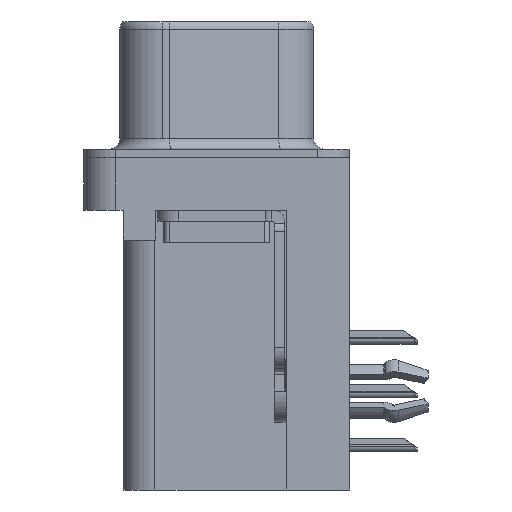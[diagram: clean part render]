
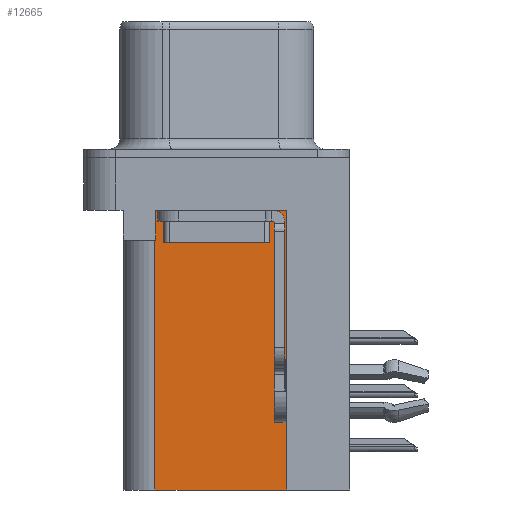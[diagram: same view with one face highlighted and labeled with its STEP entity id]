
A CAD part, left-side view. The second image highlights one B-rep face of the part: STEP entity #12665.
In plain terms, the highlighted planar face has unit normal (-1, 0, 0).
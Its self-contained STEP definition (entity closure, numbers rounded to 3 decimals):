
#93 = VECTOR ( 'NONE', #17923, 1000. ) ;
#314 = DIRECTION ( 'NONE',  ( 0., 0., 1. ) ) ;
#1641 = CARTESIAN_POINT ( 'NONE',  ( 3.7, 2.895, -3.9 ) ) ;
#2172 = VERTEX_POINT ( 'NONE', #4198 ) ;
#2786 = EDGE_CURVE ( 'NONE', #2172, #5257, #12546, .T. ) ;
#2796 = VECTOR ( 'NONE', #14160, 1000. ) ;
#2877 = LINE ( 'NONE', #1641, #2796 ) ;
#3322 = EDGE_CURVE ( 'NONE', #7064, #2172, #9905, .T. ) ;
#3385 = EDGE_CURVE ( 'NONE', #7064, #19916, #9599, .T. ) ;
#4198 = CARTESIAN_POINT ( 'NONE',  ( 3.7, 2.925, -15.7 ) ) ;
#4380 = DIRECTION ( 'NONE',  ( 0., 1., 0. ) ) ;
#5216 = ORIENTED_EDGE ( 'NONE', *, *, #24734, .T. ) ;
#5257 = VERTEX_POINT ( 'NONE', #14286 ) ;
#5856 = FACE_OUTER_BOUND ( 'NONE', #13048, .T. ) ;
#7064 = VERTEX_POINT ( 'NONE', #27423 ) ;
#9599 = LINE ( 'NONE', #19810, #9662 ) ;
#9662 = VECTOR ( 'NONE', #314, 1000. ) ;
#9745 = VECTOR ( 'NONE', #4380, 1000. ) ;
#9905 = LINE ( 'NONE', #25027, #9745 ) ;
#11982 = VECTOR ( 'NONE', #12486, 1000. ) ;
#12486 = DIRECTION ( 'NONE',  ( 0., 1., 0. ) ) ;
#12515 = VECTOR ( 'NONE', #23808, 1000. ) ;
#12546 = LINE ( 'NONE', #25858, #12515 ) ;
#12619 = LINE ( 'NONE', #17079, #11982 ) ;
#12665 = ADVANCED_FACE ( 'NONE', ( #5856 ), #21833, .F. ) ;
#13048 = EDGE_LOOP ( 'NONE', ( #30845, #30718, #5216, #14829, #28583, #13644 ) ) ;
#13597 = LINE ( 'NONE', #15676, #93 ) ;
#13644 = ORIENTED_EDGE ( 'NONE', *, *, #3385, .T. ) ;
#13768 = CARTESIAN_POINT ( 'NONE',  ( 3.7, -3.295, -2.5 ) ) ;
#14160 = DIRECTION ( 'NONE',  ( 0., 0., -1. ) ) ;
#14286 = CARTESIAN_POINT ( 'NONE',  ( 3.7, 2.925, -3.9 ) ) ;
#14829 = ORIENTED_EDGE ( 'NONE', *, *, #2786, .F. ) ;
#14872 = CARTESIAN_POINT ( 'NONE',  ( 3.7, -3.295, -15.7 ) ) ;
#15676 = CARTESIAN_POINT ( 'NONE',  ( 3.7, 0., -3.9 ) ) ;
#16013 = VERTEX_POINT ( 'NONE', #27920 ) ;
#17079 = CARTESIAN_POINT ( 'NONE',  ( 3.7, -3.295, -2.5 ) ) ;
#17171 = DIRECTION ( 'NONE',  ( 0., 0., -1. ) ) ;
#17923 = DIRECTION ( 'NONE',  ( 0., 1., 0. ) ) ;
#18250 = VERTEX_POINT ( 'NONE', #21418 ) ;
#18843 = EDGE_CURVE ( 'NONE', #19916, #18250, #12619, .T. ) ;
#19810 = CARTESIAN_POINT ( 'NONE',  ( 3.7, -3.295, -15.7 ) ) ;
#19916 = VERTEX_POINT ( 'NONE', #13768 ) ;
#19984 = EDGE_CURVE ( 'NONE', #18250, #16013, #2877, .T. ) ;
#21418 = CARTESIAN_POINT ( 'NONE',  ( 3.7, 2.895, -2.5 ) ) ;
#21833 = PLANE ( 'NONE',  #22133 ) ;
#22133 = AXIS2_PLACEMENT_3D ( 'NONE', #14872, #31141, #17171 ) ;
#23808 = DIRECTION ( 'NONE',  ( 0., 0., 1. ) ) ;
#24734 = EDGE_CURVE ( 'NONE', #16013, #5257, #13597, .T. ) ;
#25027 = CARTESIAN_POINT ( 'NONE',  ( 3.7, -3.295, -15.7 ) ) ;
#25858 = CARTESIAN_POINT ( 'NONE',  ( 3.7, 2.925, -15.7 ) ) ;
#27423 = CARTESIAN_POINT ( 'NONE',  ( 3.7, -3.295, -15.7 ) ) ;
#27920 = CARTESIAN_POINT ( 'NONE',  ( 3.7, 2.895, -3.9 ) ) ;
#28583 = ORIENTED_EDGE ( 'NONE', *, *, #3322, .F. ) ;
#30718 = ORIENTED_EDGE ( 'NONE', *, *, #19984, .T. ) ;
#30845 = ORIENTED_EDGE ( 'NONE', *, *, #18843, .T. ) ;
#31141 = DIRECTION ( 'NONE',  ( 1., 0., 0. ) ) ;
